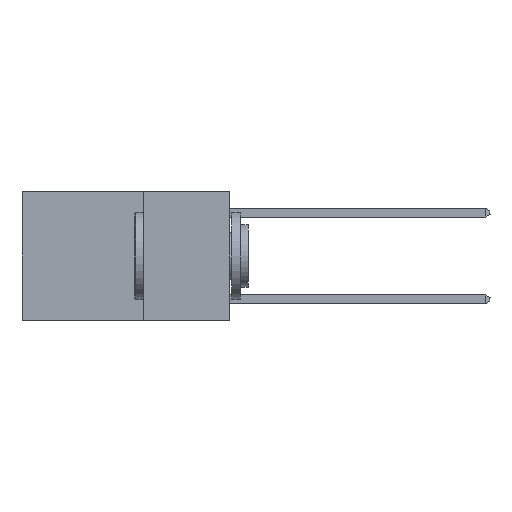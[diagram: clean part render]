
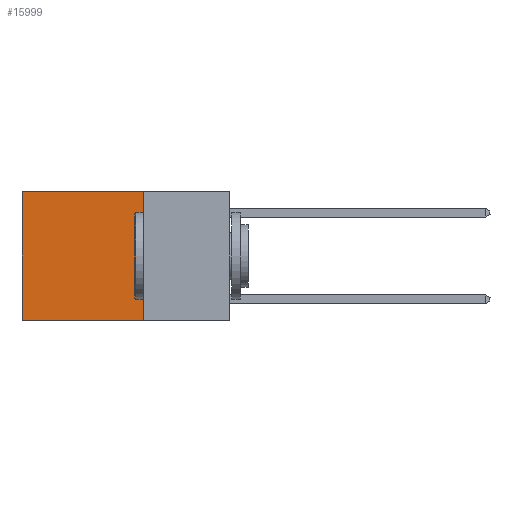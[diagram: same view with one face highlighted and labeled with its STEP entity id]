
A CAD part, left-side view. The second image highlights one B-rep face of the part: STEP entity #15999.
In plain terms, the highlighted planar face has unit normal (-1, 0, 0).
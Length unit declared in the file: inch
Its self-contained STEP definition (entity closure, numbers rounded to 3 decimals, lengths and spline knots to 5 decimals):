
#543 = PLANE ( 'NONE',  #11693 ) ;
#598 = EDGE_CURVE ( 'NONE', #7697, #11929, #10781, .T. ) ;
#622 = DIRECTION ( 'NONE',  ( 0., 0., -1. ) ) ;
#995 = ORIENTED_EDGE ( 'NONE', *, *, #15199, .F. ) ;
#1321 = EDGE_CURVE ( 'NONE', #7697, #4653, #2702, .T. ) ;
#2229 = DIRECTION ( 'NONE',  ( 0., 0., -1. ) ) ;
#2702 = LINE ( 'NONE', #8983, #16012 ) ;
#3099 = CARTESIAN_POINT ( 'NONE',  ( 0.2625, 0.25, 0. ) ) ;
#3666 = CARTESIAN_POINT ( 'NONE',  ( 0.2625, 0.6, 0. ) ) ;
#4023 = EDGE_CURVE ( 'NONE', #4653, #7883, #6161, .T. ) ;
#4653 = VERTEX_POINT ( 'NONE', #10275 ) ;
#4916 = DIRECTION ( 'NONE',  ( 0., 1., 0. ) ) ;
#5139 = CARTESIAN_POINT ( 'NONE',  ( 0.2625, 0.6, -0.37 ) ) ;
#6161 = LINE ( 'NONE', #3666, #9049 ) ;
#7697 = VERTEX_POINT ( 'NONE', #11753 ) ;
#7883 = VERTEX_POINT ( 'NONE', #5139 ) ;
#8060 = DIRECTION ( 'NONE',  ( 1., 0., 0. ) ) ;
#8983 = CARTESIAN_POINT ( 'NONE',  ( 0.2625, 0.25, 0. ) ) ;
#9049 = VECTOR ( 'NONE', #16000, 39.37008 ) ;
#9481 = VECTOR ( 'NONE', #2229, 39.37008 ) ;
#10275 = CARTESIAN_POINT ( 'NONE',  ( 0.2625, 0.6, 0. ) ) ;
#10781 = LINE ( 'NONE', #13380, #9481 ) ;
#11693 = AXIS2_PLACEMENT_3D ( 'NONE', #3099, #8060, #622 ) ;
#11753 = CARTESIAN_POINT ( 'NONE',  ( 0.2625, 0.25, 0. ) ) ;
#11864 = DIRECTION ( 'NONE',  ( 0., 1., 0. ) ) ;
#11929 = VERTEX_POINT ( 'NONE', #13185 ) ;
#12463 = ORIENTED_EDGE ( 'NONE', *, *, #1321, .T. ) ;
#12984 = VECTOR ( 'NONE', #4916, 39.37008 ) ;
#12990 = ORIENTED_EDGE ( 'NONE', *, *, #4023, .T. ) ;
#13185 = CARTESIAN_POINT ( 'NONE',  ( 0.2625, 0.25, -0.37 ) ) ;
#13380 = CARTESIAN_POINT ( 'NONE',  ( 0.2625, 0.25, 0. ) ) ;
#14738 = LINE ( 'NONE', #16050, #12984 ) ;
#15199 = EDGE_CURVE ( 'NONE', #11929, #7883, #14738, .T. ) ;
#15610 = FACE_OUTER_BOUND ( 'NONE', #15910, .T. ) ;
#15666 = ORIENTED_EDGE ( 'NONE', *, *, #598, .F. ) ;
#15910 = EDGE_LOOP ( 'NONE', ( #12990, #995, #15666, #12463 ) ) ;
#15999 = ADVANCED_FACE ( 'NONE', ( #15610 ), #543, .F. ) ;
#16000 = DIRECTION ( 'NONE',  ( 0., 0., -1. ) ) ;
#16012 = VECTOR ( 'NONE', #11864, 39.37008 ) ;
#16050 = CARTESIAN_POINT ( 'NONE',  ( 0.2625, 0.25, -0.37 ) ) ;
